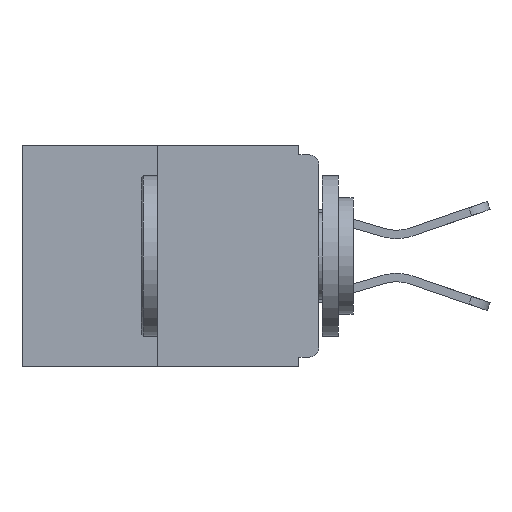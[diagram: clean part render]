
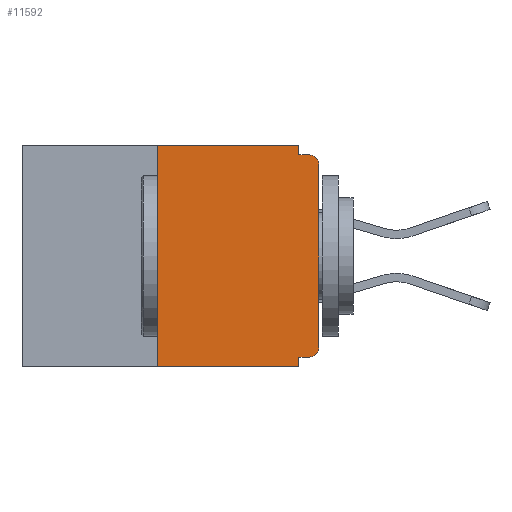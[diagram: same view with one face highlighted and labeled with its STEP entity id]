
A CAD part, left-side view. The second image highlights one B-rep face of the part: STEP entity #11592.
In plain terms, the highlighted planar face has unit normal (-1, 0, 0).
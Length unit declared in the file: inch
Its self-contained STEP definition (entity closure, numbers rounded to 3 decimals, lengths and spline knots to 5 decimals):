
#86 = CARTESIAN_POINT ( 'NONE',  ( 0., 0.031, 0. ) ) ;
#292 = CARTESIAN_POINT ( 'NONE',  ( 0., 0.25, -0.343 ) ) ;
#430 = EDGE_CURVE ( 'NONE', #12091, #7273, #2973, .T. ) ;
#704 = EDGE_CURVE ( 'NONE', #6297, #11374, #2821, .T. ) ;
#1242 = VECTOR ( 'NONE', #7159, 39.37008 ) ;
#1413 = EDGE_LOOP ( 'NONE', ( #9521, #1884, #7958, #7307, #5964, #9093, #4012, #7267, #7810, #8280 ) ) ;
#1468 = DIRECTION ( 'NONE',  ( 0., 0., 1. ) ) ;
#1884 = ORIENTED_EDGE ( 'NONE', *, *, #704, .F. ) ;
#1919 = LINE ( 'NONE', #2261, #12504 ) ;
#2067 = DIRECTION ( 'NONE',  ( 1., 0., 0. ) ) ;
#2230 = VERTEX_POINT ( 'NONE', #7240 ) ;
#2261 = CARTESIAN_POINT ( 'NONE',  ( 0., 0.031, 0. ) ) ;
#2395 = VERTEX_POINT ( 'NONE', #86 ) ;
#2398 = DIRECTION ( 'NONE',  ( 0., 0., -1. ) ) ;
#2604 = FACE_OUTER_BOUND ( 'NONE', #1413, .T. ) ;
#2821 = LINE ( 'NONE', #7757, #9570 ) ;
#2973 = LINE ( 'NONE', #10291, #1242 ) ;
#3279 = CARTESIAN_POINT ( 'NONE',  ( 0., 0.031, -0.343 ) ) ;
#3546 = DIRECTION ( 'NONE',  ( -1., 0., 0. ) ) ;
#3594 = LINE ( 'NONE', #5923, #13090 ) ;
#3650 = DIRECTION ( 'NONE',  ( 0., 0., -1. ) ) ;
#3713 = VECTOR ( 'NONE', #8314, 39.37008 ) ;
#4012 = ORIENTED_EDGE ( 'NONE', *, *, #6784, .T. ) ;
#4061 = CARTESIAN_POINT ( 'NONE',  ( 0., 0.031, -0.343 ) ) ;
#4693 = DIRECTION ( 'NONE',  ( 0., -1., 0. ) ) ;
#4823 = AXIS2_PLACEMENT_3D ( 'NONE', #8461, #12523, #12439 ) ;
#4854 = LINE ( 'NONE', #12878, #5314 ) ;
#5300 = CARTESIAN_POINT ( 'NONE',  ( 0., 0., -0.313 ) ) ;
#5314 = VECTOR ( 'NONE', #6658, 39.37008 ) ;
#5375 = VERTEX_POINT ( 'NONE', #10524 ) ;
#5669 = EDGE_CURVE ( 'NONE', #12735, #5375, #6347, .T. ) ;
#5701 = LINE ( 'NONE', #3279, #10125 ) ;
#5923 = CARTESIAN_POINT ( 'NONE',  ( 0., 0.46, 0. ) ) ;
#5964 = ORIENTED_EDGE ( 'NONE', *, *, #430, .F. ) ;
#6066 = CARTESIAN_POINT ( 'NONE',  ( 0., 0.46, 0. ) ) ;
#6297 = VERTEX_POINT ( 'NONE', #292 ) ;
#6347 = CIRCLE ( 'NONE', #9375, 0.015 ) ;
#6658 = DIRECTION ( 'NONE',  ( 0., -1., 0. ) ) ;
#6784 = EDGE_CURVE ( 'NONE', #8950, #12735, #12117, .T. ) ;
#7159 = DIRECTION ( 'NONE',  ( 0., 1., 0. ) ) ;
#7240 = CARTESIAN_POINT ( 'NONE',  ( 0., 0.031, -0.015 ) ) ;
#7267 = ORIENTED_EDGE ( 'NONE', *, *, #5669, .T. ) ;
#7273 = VERTEX_POINT ( 'NONE', #8691 ) ;
#7307 = ORIENTED_EDGE ( 'NONE', *, *, #12939, .F. ) ;
#7492 = DIRECTION ( 'NONE',  ( 0., 0., 1. ) ) ;
#7618 = EDGE_CURVE ( 'NONE', #6297, #13459, #4854, .T. ) ;
#7757 = CARTESIAN_POINT ( 'NONE',  ( 0., 0.25, 0. ) ) ;
#7791 = CARTESIAN_POINT ( 'NONE',  ( 0., 0.25, 0. ) ) ;
#7810 = ORIENTED_EDGE ( 'NONE', *, *, #12685, .F. ) ;
#7958 = ORIENTED_EDGE ( 'NONE', *, *, #7618, .T. ) ;
#8280 = ORIENTED_EDGE ( 'NONE', *, *, #13068, .F. ) ;
#8314 = DIRECTION ( 'NONE',  ( 0., -1., 0. ) ) ;
#8374 = CARTESIAN_POINT ( 'NONE',  ( 0., 0., 0. ) ) ;
#8461 = CARTESIAN_POINT ( 'NONE',  ( 0., 0.015, -0.313 ) ) ;
#8691 = CARTESIAN_POINT ( 'NONE',  ( 0., 0.031, -0.328 ) ) ;
#8737 = CIRCLE ( 'NONE', #4823, 0.015 ) ;
#8950 = VERTEX_POINT ( 'NONE', #5300 ) ;
#9093 = ORIENTED_EDGE ( 'NONE', *, *, #13536, .T. ) ;
#9358 = VECTOR ( 'NONE', #7492, 39.37008 ) ;
#9375 = AXIS2_PLACEMENT_3D ( 'NONE', #9858, #3546, #3650 ) ;
#9458 = CARTESIAN_POINT ( 'NONE',  ( 0., 0., -0.015 ) ) ;
#9521 = ORIENTED_EDGE ( 'NONE', *, *, #11418, .F. ) ;
#9570 = VECTOR ( 'NONE', #1468, 39.37008 ) ;
#9832 = DIRECTION ( 'NONE',  ( 0., 0., -1. ) ) ;
#9858 = CARTESIAN_POINT ( 'NONE',  ( 0., 0.015, -0.03 ) ) ;
#10125 = VECTOR ( 'NONE', #9832, 39.37008 ) ;
#10220 = AXIS2_PLACEMENT_3D ( 'NONE', #6066, #2067, #10755 ) ;
#10282 = LINE ( 'NONE', #9458, #3713 ) ;
#10291 = CARTESIAN_POINT ( 'NONE',  ( 0., 0., -0.328 ) ) ;
#10524 = CARTESIAN_POINT ( 'NONE',  ( 0., 0.015, -0.015 ) ) ;
#10755 = DIRECTION ( 'NONE',  ( 0., 0., -1. ) ) ;
#11374 = VERTEX_POINT ( 'NONE', #7791 ) ;
#11418 = EDGE_CURVE ( 'NONE', #11374, #2395, #3594, .T. ) ;
#11592 = ADVANCED_FACE ( 'NONE', ( #2604 ), #12086, .F. ) ;
#12086 = PLANE ( 'NONE',  #10220 ) ;
#12091 = VERTEX_POINT ( 'NONE', #13487 ) ;
#12117 = LINE ( 'NONE', #8374, #9358 ) ;
#12439 = DIRECTION ( 'NONE',  ( 0., 0., -1. ) ) ;
#12504 = VECTOR ( 'NONE', #2398, 39.37008 ) ;
#12523 = DIRECTION ( 'NONE',  ( -1., 0., 0. ) ) ;
#12571 = CARTESIAN_POINT ( 'NONE',  ( 0., 0., -0.03 ) ) ;
#12685 = EDGE_CURVE ( 'NONE', #2230, #5375, #10282, .T. ) ;
#12735 = VERTEX_POINT ( 'NONE', #12571 ) ;
#12878 = CARTESIAN_POINT ( 'NONE',  ( 0., 0.46, -0.343 ) ) ;
#12939 = EDGE_CURVE ( 'NONE', #7273, #13459, #5701, .T. ) ;
#13068 = EDGE_CURVE ( 'NONE', #2395, #2230, #1919, .T. ) ;
#13090 = VECTOR ( 'NONE', #4693, 39.37008 ) ;
#13459 = VERTEX_POINT ( 'NONE', #4061 ) ;
#13487 = CARTESIAN_POINT ( 'NONE',  ( 0., 0.015, -0.328 ) ) ;
#13536 = EDGE_CURVE ( 'NONE', #12091, #8950, #8737, .T. ) ;
